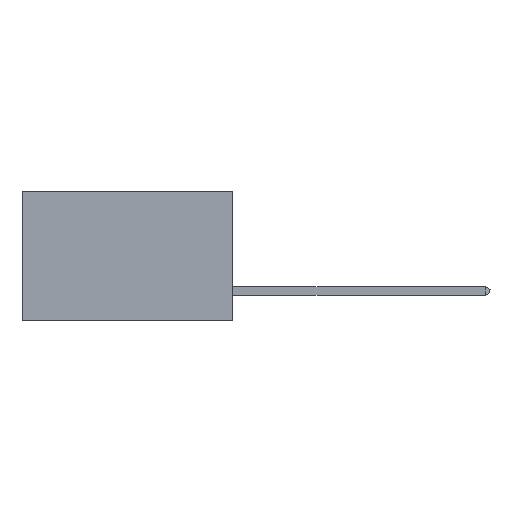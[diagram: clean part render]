
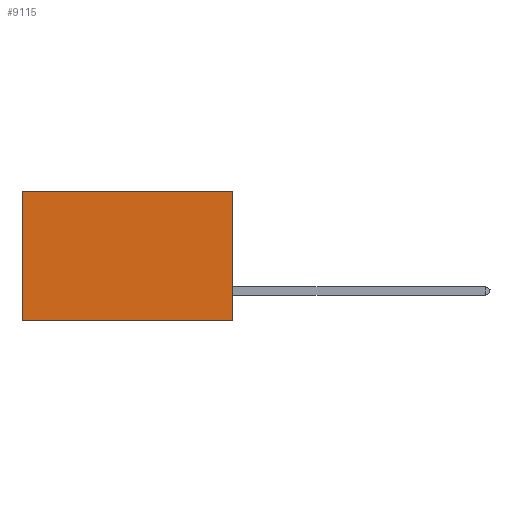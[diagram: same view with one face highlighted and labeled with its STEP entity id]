
A CAD part, left-side view. The second image highlights one B-rep face of the part: STEP entity #9115.
In plain terms, the highlighted planar face has unit normal (-1, 0, 0).
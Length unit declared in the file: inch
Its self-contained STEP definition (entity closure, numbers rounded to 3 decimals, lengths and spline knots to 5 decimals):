
#8 = CARTESIAN_POINT ( 'NONE',  ( 0.2875, 0., 0. ) ) ;
#121 = ORIENTED_EDGE ( 'NONE', *, *, #2534, .T. ) ;
#262 = DIRECTION ( 'NONE',  ( 0., 0., -1. ) ) ;
#389 = DIRECTION ( 'NONE',  ( 0., 0., -1. ) ) ;
#1952 = CARTESIAN_POINT ( 'NONE',  ( 0.2875, 0., -0.37 ) ) ;
#2534 = EDGE_CURVE ( 'NONE', #9236, #7197, #3916, .T. ) ;
#3109 = ORIENTED_EDGE ( 'NONE', *, *, #8312, .F. ) ;
#3132 = CARTESIAN_POINT ( 'NONE',  ( 0.2875, 0.6, -0.37 ) ) ;
#3495 = ORIENTED_EDGE ( 'NONE', *, *, #5435, .F. ) ;
#3861 = VECTOR ( 'NONE', #262, 39.37008 ) ;
#3916 = LINE ( 'NONE', #8, #9521 ) ;
#4315 = EDGE_LOOP ( 'NONE', ( #8402, #3109, #3495, #121 ) ) ;
#4629 = AXIS2_PLACEMENT_3D ( 'NONE', #9977, #5907, #4920 ) ;
#4920 = DIRECTION ( 'NONE',  ( 0., 0., -1. ) ) ;
#5435 = EDGE_CURVE ( 'NONE', #9236, #7835, #10053, .T. ) ;
#5508 = LINE ( 'NONE', #1952, #7537 ) ;
#5907 = DIRECTION ( 'NONE',  ( 1., 0., 0. ) ) ;
#7197 = VERTEX_POINT ( 'NONE', #7995 ) ;
#7537 = VECTOR ( 'NONE', #9890, 39.37008 ) ;
#7835 = VERTEX_POINT ( 'NONE', #12331 ) ;
#7995 = CARTESIAN_POINT ( 'NONE',  ( 0.2875, 0.6, 0. ) ) ;
#8200 = CARTESIAN_POINT ( 'NONE',  ( 0.2875, 0., 0. ) ) ;
#8312 = EDGE_CURVE ( 'NONE', #7835, #8507, #5508, .T. ) ;
#8402 = ORIENTED_EDGE ( 'NONE', *, *, #9934, .T. ) ;
#8507 = VERTEX_POINT ( 'NONE', #3132 ) ;
#9115 = ADVANCED_FACE ( 'NONE', ( #10094 ), #10945, .F. ) ;
#9236 = VERTEX_POINT ( 'NONE', #8200 ) ;
#9298 = CARTESIAN_POINT ( 'NONE',  ( 0.2875, 0.6, 0. ) ) ;
#9521 = VECTOR ( 'NONE', #9902, 39.37008 ) ;
#9890 = DIRECTION ( 'NONE',  ( 0., 1., 0. ) ) ;
#9902 = DIRECTION ( 'NONE',  ( 0., 1., 0. ) ) ;
#9934 = EDGE_CURVE ( 'NONE', #7197, #8507, #10535, .T. ) ;
#9977 = CARTESIAN_POINT ( 'NONE',  ( 0.2875, 0., 0. ) ) ;
#10053 = LINE ( 'NONE', #12066, #3861 ) ;
#10094 = FACE_OUTER_BOUND ( 'NONE', #4315, .T. ) ;
#10535 = LINE ( 'NONE', #9298, #12715 ) ;
#10945 = PLANE ( 'NONE',  #4629 ) ;
#12066 = CARTESIAN_POINT ( 'NONE',  ( 0.2875, 0., 0. ) ) ;
#12331 = CARTESIAN_POINT ( 'NONE',  ( 0.2875, 0., -0.37 ) ) ;
#12715 = VECTOR ( 'NONE', #389, 39.37008 ) ;
